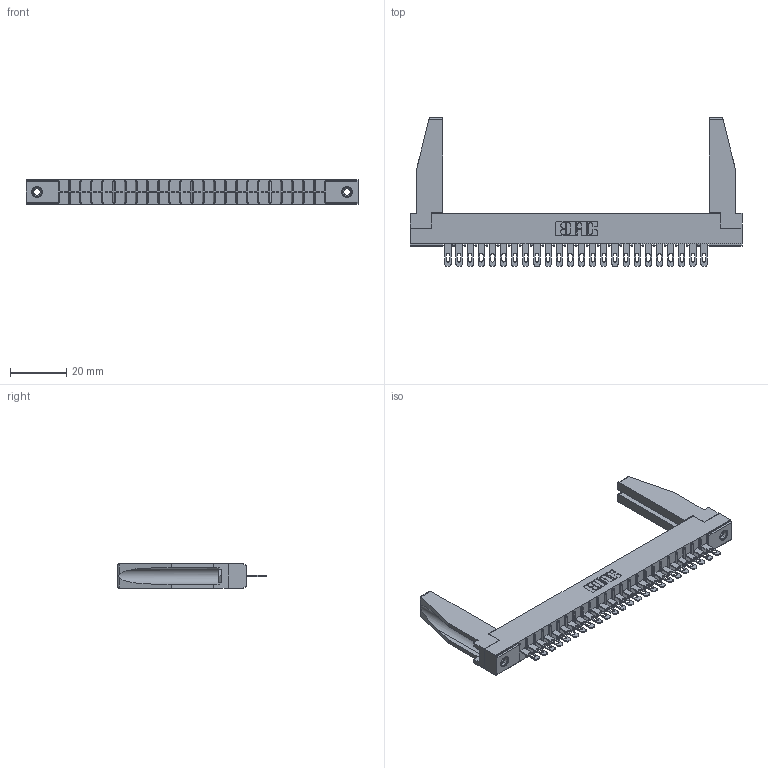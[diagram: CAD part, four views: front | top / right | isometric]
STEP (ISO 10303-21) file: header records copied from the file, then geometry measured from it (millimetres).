
FILE_DESCRIPTION (( 'STEP AP203' ), '1' );
FILE_NAME ('356-024-500-178.STEP', '2018-08-01T20:07:52', ( '' ), ( '' ), 'SwSTEP 2.0', 'SolidWorks 2016', '' );
FILE_SCHEMA (( 'CONFIG_CONTROL_DESIGN' ));
Length unit declared in the file: inch
Products named in the file (5): 307-220-078; 356-024-500-178; 306 Part_.156 Dia; 306-290-001_100; 345-250-001_345-250-001-102
Assembly tree (29 placements, depth 2):
  356-024-500-178
    306 Part_.156 Dia
    306-290-001_100  x24
    345-250-001_345-250-001-102  x2
    307-220-078  x2
Bounding box: 118.11 x 52.91 x 8.71 mm (x, y, z)
Volume: 12153.2 mm3; surface area: 16347.6 mm2
Topology: 29 solids, 29 shells, 2070 faces, 5806 edges, 3732 vertices
Faces by surface type: plane 1352, cylinder 606, sphere 96, cone 12, torus 4
Entity records: 27316 total; most frequent: CARTESIAN_POINT 4585, ORIENTED_EDGE 4502, DIRECTION 4475, EDGE_CURVE 2251, LINE 1751, VECTOR 1751, VERTEX_POINT 1430, AXIS2_PLACEMENT_3D 1362
